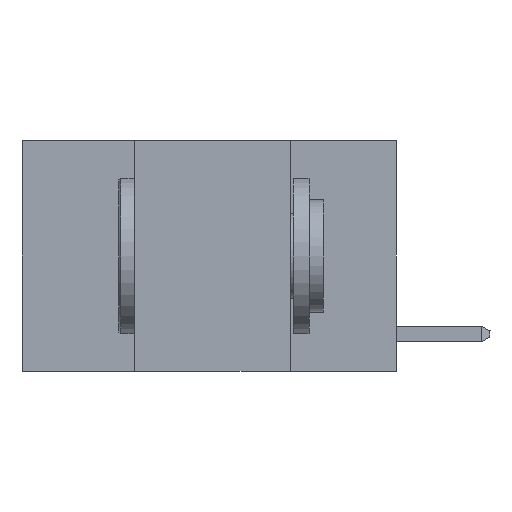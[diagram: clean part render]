
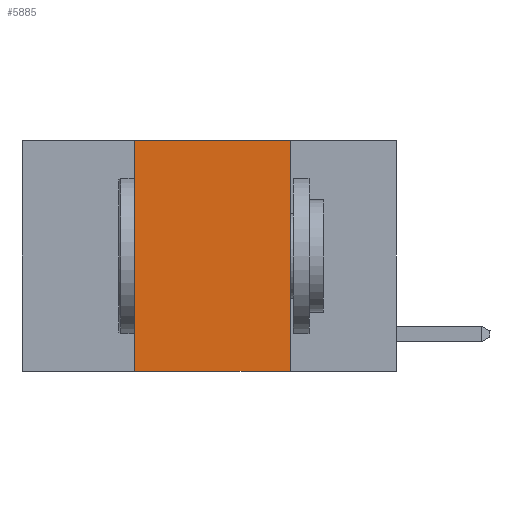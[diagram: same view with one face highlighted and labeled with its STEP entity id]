
A CAD part, left-side view. The second image highlights one B-rep face of the part: STEP entity #5885.
In plain terms, the highlighted planar face has unit normal (-1, 0, 0).
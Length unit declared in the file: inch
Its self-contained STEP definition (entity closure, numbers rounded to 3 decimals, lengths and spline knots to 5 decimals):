
#240 = VECTOR ( 'NONE', #1016, 39.37008 ) ;
#247 = CARTESIAN_POINT ( 'NONE',  ( 0., 0.6, 0. ) ) ;
#468 = LINE ( 'NONE', #628, #3868 ) ;
#628 = CARTESIAN_POINT ( 'NONE',  ( 0., 0.17, 0. ) ) ;
#1016 = DIRECTION ( 'NONE',  ( 0., -1., 0. ) ) ;
#1809 = ORIENTED_EDGE ( 'NONE', *, *, #2864, .T. ) ;
#2048 = EDGE_CURVE ( 'NONE', #11467, #2290, #2682, .T. ) ;
#2290 = VERTEX_POINT ( 'NONE', #5900 ) ;
#2404 = EDGE_LOOP ( 'NONE', ( #10785, #3888, #10207, #1809 ) ) ;
#2682 = LINE ( 'NONE', #247, #9938 ) ;
#2864 = EDGE_CURVE ( 'NONE', #10140, #8155, #7968, .T. ) ;
#2865 = DIRECTION ( 'NONE',  ( 0., 0., 1. ) ) ;
#3186 = DIRECTION ( 'NONE',  ( 1., 0., 0. ) ) ;
#3668 = LINE ( 'NONE', #4667, #4244 ) ;
#3868 = VECTOR ( 'NONE', #9170, 39.37008 ) ;
#3888 = ORIENTED_EDGE ( 'NONE', *, *, #2048, .F. ) ;
#4244 = VECTOR ( 'NONE', #2865, 39.37008 ) ;
#4667 = CARTESIAN_POINT ( 'NONE',  ( 0., 0.42, 0. ) ) ;
#5635 = CARTESIAN_POINT ( 'NONE',  ( 0., 0.6, -0.37 ) ) ;
#5727 = EDGE_CURVE ( 'NONE', #2290, #8155, #468, .T. ) ;
#5885 = ADVANCED_FACE ( 'NONE', ( #11448 ), #8883, .F. ) ;
#5900 = CARTESIAN_POINT ( 'NONE',  ( 0., 0.17, 0. ) ) ;
#5959 = CARTESIAN_POINT ( 'NONE',  ( 0., 0.6, 0. ) ) ;
#6076 = AXIS2_PLACEMENT_3D ( 'NONE', #5959, #3186, #10791 ) ;
#6953 = DIRECTION ( 'NONE',  ( 0., -1., 0. ) ) ;
#7170 = CARTESIAN_POINT ( 'NONE',  ( 0., 0.42, -0.37 ) ) ;
#7968 = LINE ( 'NONE', #5635, #240 ) ;
#8021 = EDGE_CURVE ( 'NONE', #10140, #11467, #3668, .T. ) ;
#8155 = VERTEX_POINT ( 'NONE', #10526 ) ;
#8883 = PLANE ( 'NONE',  #6076 ) ;
#9170 = DIRECTION ( 'NONE',  ( 0., 0., -1. ) ) ;
#9938 = VECTOR ( 'NONE', #6953, 39.37008 ) ;
#10140 = VERTEX_POINT ( 'NONE', #7170 ) ;
#10207 = ORIENTED_EDGE ( 'NONE', *, *, #8021, .F. ) ;
#10526 = CARTESIAN_POINT ( 'NONE',  ( 0., 0.17, -0.37 ) ) ;
#10700 = CARTESIAN_POINT ( 'NONE',  ( 0., 0.42, 0. ) ) ;
#10785 = ORIENTED_EDGE ( 'NONE', *, *, #5727, .F. ) ;
#10791 = DIRECTION ( 'NONE',  ( 0., 0., -1. ) ) ;
#11448 = FACE_OUTER_BOUND ( 'NONE', #2404, .T. ) ;
#11467 = VERTEX_POINT ( 'NONE', #10700 ) ;
